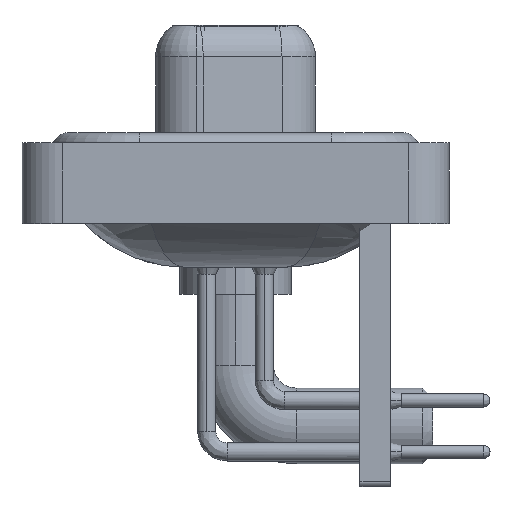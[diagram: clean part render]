
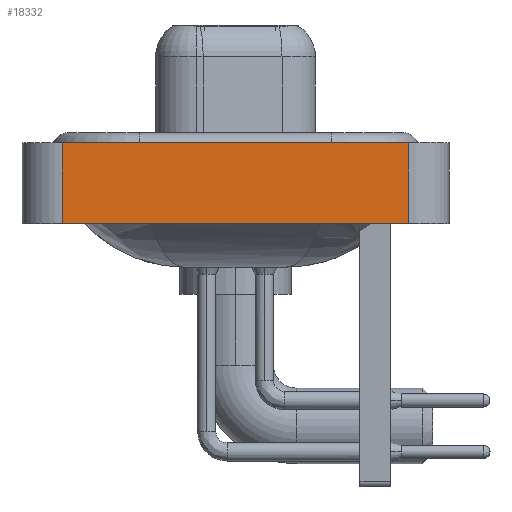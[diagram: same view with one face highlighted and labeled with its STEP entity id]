
A CAD part, left-side view. The second image highlights one B-rep face of the part: STEP entity #18332.
In plain terms, the highlighted planar face has unit normal (-1, 0, 0).
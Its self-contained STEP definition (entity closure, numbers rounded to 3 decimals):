
#62 = CARTESIAN_POINT ( 'NONE',  ( -7.35, -8.55, -3.6 ) ) ;
#590 = VERTEX_POINT ( 'NONE', #22292 ) ;
#1445 = DIRECTION ( 'NONE',  ( 0., 0., 1. ) ) ;
#1645 = CARTESIAN_POINT ( 'NONE',  ( -7.35, -8.55, -3.6 ) ) ;
#2460 = CARTESIAN_POINT ( 'NONE',  ( -7.35, -8.55, 0.4 ) ) ;
#2993 = CARTESIAN_POINT ( 'NONE',  ( -7.35, -8.55, 0.4 ) ) ;
#4065 = VERTEX_POINT ( 'NONE', #62 ) ;
#5307 = LINE ( 'NONE', #22092, #18769 ) ;
#5782 = ORIENTED_EDGE ( 'NONE', *, *, #26202, .T. ) ;
#6505 = FACE_OUTER_BOUND ( 'NONE', #17175, .T. ) ;
#8766 = LINE ( 'NONE', #21576, #27106 ) ;
#8832 = VERTEX_POINT ( 'NONE', #2993 ) ;
#8894 = LINE ( 'NONE', #2460, #22659 ) ;
#10447 = ORIENTED_EDGE ( 'NONE', *, *, #11536, .F. ) ;
#10773 = DIRECTION ( 'NONE',  ( 0., 0., 1. ) ) ;
#11536 = EDGE_CURVE ( 'NONE', #590, #8832, #8894, .T. ) ;
#11935 = EDGE_CURVE ( 'NONE', #17379, #590, #8766, .T. ) ;
#12656 = ORIENTED_EDGE ( 'NONE', *, *, #23096, .T. ) ;
#15026 = PLANE ( 'NONE',  #21282 ) ;
#15309 = DIRECTION ( 'NONE',  ( -1., 0., 0. ) ) ;
#15382 = DIRECTION ( 'NONE',  ( 0., -1., 0. ) ) ;
#15700 = DIRECTION ( 'NONE',  ( 0., -1., 0. ) ) ;
#17175 = EDGE_LOOP ( 'NONE', ( #5782, #10447, #26219, #12656 ) ) ;
#17329 = DIRECTION ( 'NONE',  ( 0., 0., 1. ) ) ;
#17379 = VERTEX_POINT ( 'NONE', #19250 ) ;
#18332 = ADVANCED_FACE ( 'NONE', ( #6505 ), #15026, .T. ) ;
#18769 = VECTOR ( 'NONE', #1445, 1000. ) ;
#19250 = CARTESIAN_POINT ( 'NONE',  ( -7.35, 8.55, -3.6 ) ) ;
#21282 = AXIS2_PLACEMENT_3D ( 'NONE', #25479, #15309, #10773 ) ;
#21576 = CARTESIAN_POINT ( 'NONE',  ( -7.35, 8.55, -3.6 ) ) ;
#22092 = CARTESIAN_POINT ( 'NONE',  ( -7.35, -8.55, -3.6 ) ) ;
#22292 = CARTESIAN_POINT ( 'NONE',  ( -7.35, 8.55, 0.4 ) ) ;
#22659 = VECTOR ( 'NONE', #15382, 1000. ) ;
#23096 = EDGE_CURVE ( 'NONE', #17379, #4065, #24484, .T. ) ;
#24484 = LINE ( 'NONE', #1645, #25360 ) ;
#25360 = VECTOR ( 'NONE', #15700, 1000. ) ;
#25479 = CARTESIAN_POINT ( 'NONE',  ( -7.35, -8.55, -3.6 ) ) ;
#26202 = EDGE_CURVE ( 'NONE', #4065, #8832, #5307, .T. ) ;
#26219 = ORIENTED_EDGE ( 'NONE', *, *, #11935, .F. ) ;
#27106 = VECTOR ( 'NONE', #17329, 1000. ) ;
